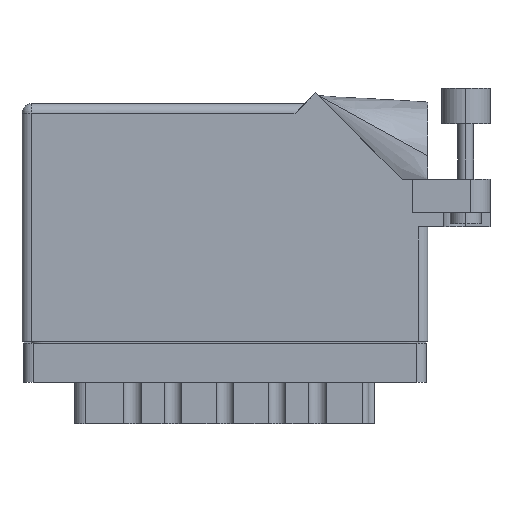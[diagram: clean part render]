
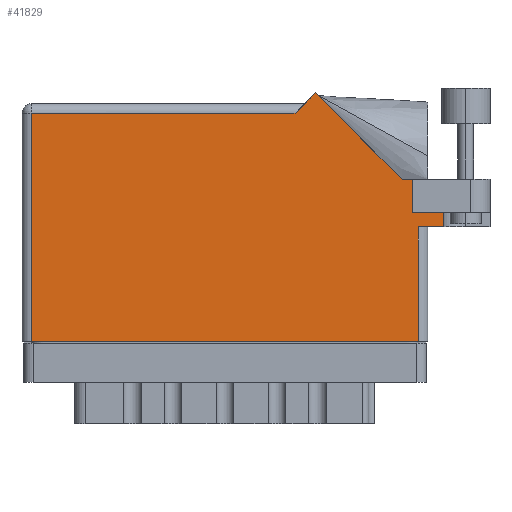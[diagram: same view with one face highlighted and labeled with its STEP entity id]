
A CAD part, front view. The second image highlights one B-rep face of the part: STEP entity #41829.
In plain terms, the highlighted face is planar.
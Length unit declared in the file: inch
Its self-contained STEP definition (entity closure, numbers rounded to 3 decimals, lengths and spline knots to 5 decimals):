
#78 = DIRECTION ( 'NONE',  ( 0., 1., 0. ) ) ;
#1935 = LINE ( 'NONE', #53545, #23391 ) ;
#1975 = LINE ( 'NONE', #14312, #14341 ) ;
#2028 = LINE ( 'NONE', #33242, #18279 ) ;
#2442 = DIRECTION ( 'NONE',  ( -0.707, -0.707, 0. ) ) ;
#4687 = PLANE ( 'NONE',  #38663 ) ;
#5267 = CARTESIAN_POINT ( 'NONE',  ( 0., 1.468, 0. ) ) ;
#6086 = ORIENTED_EDGE ( 'NONE', *, *, #46386, .T. ) ;
#6422 = EDGE_CURVE ( 'NONE', #45393, #26172, #22502, .T. ) ;
#6703 = VERTEX_POINT ( 'NONE', #28338 ) ;
#7091 = DIRECTION ( 'NONE',  ( 0., -1., 0. ) ) ;
#8161 = CARTESIAN_POINT ( 'NONE',  ( 0., 0., 0. ) ) ;
#8495 = DIRECTION ( 'NONE',  ( -1., 0., 0. ) ) ;
#11609 = CARTESIAN_POINT ( 'NONE',  ( 2.7135, 1.16177, 0. ) ) ;
#12663 = CARTESIAN_POINT ( 'NONE',  ( 0., 1.53, 0. ) ) ;
#12976 = CARTESIAN_POINT ( 'NONE',  ( 0.062, 0., 0. ) ) ;
#13399 = ORIENTED_EDGE ( 'NONE', *, *, #14437, .F. ) ;
#14090 = VECTOR ( 'NONE', #7091, 39.37008 ) ;
#14312 = CARTESIAN_POINT ( 'NONE',  ( 0.062, 0., 0. ) ) ;
#14341 = VECTOR ( 'NONE', #22461, 39.37008 ) ;
#14437 = EDGE_CURVE ( 'NONE', #32994, #45393, #21769, .T. ) ;
#14681 = CARTESIAN_POINT ( 'NONE',  ( 2.512, 0.831, 0. ) ) ;
#14711 = VECTOR ( 'NONE', #39301, 39.37008 ) ;
#15685 = VECTOR ( 'NONE', #33234, 39.37008 ) ;
#16981 = LINE ( 'NONE', #8161, #15685 ) ;
#17054 = DIRECTION ( 'NONE',  ( -1., 0., 0. ) ) ;
#18279 = VECTOR ( 'NONE', #49422, 39.37008 ) ;
#18622 = VECTOR ( 'NONE', #78, 39.37008 ) ;
#18752 = CARTESIAN_POINT ( 'NONE',  ( 2.512, 1.044, 0. ) ) ;
#21435 = CARTESIAN_POINT ( 'NONE',  ( 2.44642, 1.044, 0. ) ) ;
#21507 = EDGE_CURVE ( 'NONE', #52375, #6703, #31253, .T. ) ;
#21769 = LINE ( 'NONE', #46541, #53081 ) ;
#22461 = DIRECTION ( 'NONE',  ( 0., -1., 0. ) ) ;
#22496 = VERTEX_POINT ( 'NONE', #32623 ) ;
#22502 = LINE ( 'NONE', #11609, #14090 ) ;
#22511 = LINE ( 'NONE', #37193, #18622 ) ;
#23029 = FACE_OUTER_BOUND ( 'NONE', #51310, .T. ) ;
#23140 = ORIENTED_EDGE ( 'NONE', *, *, #25899, .T. ) ;
#23391 = VECTOR ( 'NONE', #2442, 39.37008 ) ;
#23693 = CARTESIAN_POINT ( 'NONE',  ( 2.7135, 0.831, 0. ) ) ;
#23819 = CARTESIAN_POINT ( 'NONE',  ( 2.44642, 1.044, 0. ) ) ;
#23852 = CARTESIAN_POINT ( 'NONE',  ( 1.757, 1.468, 0. ) ) ;
#24695 = CARTESIAN_POINT ( 'NONE',  ( 2.55, 0.737, 0. ) ) ;
#24948 = VERTEX_POINT ( 'NONE', #24695 ) ;
#25200 = DIRECTION ( 'NONE',  ( 0., 0., -1. ) ) ;
#25675 = VECTOR ( 'NONE', #35914, 39.37008 ) ;
#25816 = VERTEX_POINT ( 'NONE', #39876 ) ;
#25899 = EDGE_CURVE ( 'NONE', #26541, #31645, #38672, .T. ) ;
#26172 = VERTEX_POINT ( 'NONE', #37884 ) ;
#26541 = VERTEX_POINT ( 'NONE', #18752 ) ;
#26849 = ORIENTED_EDGE ( 'NONE', *, *, #43912, .T. ) ;
#26880 = EDGE_CURVE ( 'NONE', #31645, #22496, #49626, .T. ) ;
#27528 = ORIENTED_EDGE ( 'NONE', *, *, #6422, .F. ) ;
#28338 = CARTESIAN_POINT ( 'NONE',  ( 0.062, 1.468, 0. ) ) ;
#28623 = VECTOR ( 'NONE', #17054, 39.37008 ) ;
#29414 = VECTOR ( 'NONE', #29619, 39.37008 ) ;
#29619 = DIRECTION ( 'NONE',  ( -0.707, 0.707, 0. ) ) ;
#31253 = LINE ( 'NONE', #5267, #28623 ) ;
#31645 = VERTEX_POINT ( 'NONE', #23819 ) ;
#32078 = ORIENTED_EDGE ( 'NONE', *, *, #37464, .T. ) ;
#32623 = CARTESIAN_POINT ( 'NONE',  ( 1.88971, 1.60071, 0. ) ) ;
#32932 = LINE ( 'NONE', #46960, #14711 ) ;
#32994 = VERTEX_POINT ( 'NONE', #14681 ) ;
#33209 = EDGE_CURVE ( 'NONE', #32994, #26541, #22511, .T. ) ;
#33234 = DIRECTION ( 'NONE',  ( 1., 0., 0. ) ) ;
#33242 = CARTESIAN_POINT ( 'NONE',  ( 2.55, 0.737, 0. ) ) ;
#33291 = DIRECTION ( 'NONE',  ( 1., 0., 0. ) ) ;
#34395 = ORIENTED_EDGE ( 'NONE', *, *, #43591, .T. ) ;
#35914 = DIRECTION ( 'NONE',  ( -1., 0., 0. ) ) ;
#37193 = CARTESIAN_POINT ( 'NONE',  ( 2.512, 0.831, 0. ) ) ;
#37434 = ORIENTED_EDGE ( 'NONE', *, *, #53587, .T. ) ;
#37464 = EDGE_CURVE ( 'NONE', #22496, #52375, #1935, .T. ) ;
#37884 = CARTESIAN_POINT ( 'NONE',  ( 2.7135, 0.737, 0. ) ) ;
#38266 = ORIENTED_EDGE ( 'NONE', *, *, #33209, .T. ) ;
#38663 = AXIS2_PLACEMENT_3D ( 'NONE', #12663, #25200, #8495 ) ;
#38672 = LINE ( 'NONE', #40570, #25675 ) ;
#39301 = DIRECTION ( 'NONE',  ( 1., 0., 0. ) ) ;
#39876 = CARTESIAN_POINT ( 'NONE',  ( 2.55, 0., 0. ) ) ;
#40570 = CARTESIAN_POINT ( 'NONE',  ( 3.012, 1.044, 0. ) ) ;
#41829 = ADVANCED_FACE ( 'NONE', ( #23029 ), #4687, .F. ) ;
#42380 = VERTEX_POINT ( 'NONE', #12976 ) ;
#43591 = EDGE_CURVE ( 'NONE', #25816, #24948, #2028, .T. ) ;
#43912 = EDGE_CURVE ( 'NONE', #6703, #42380, #1975, .T. ) ;
#44953 = ORIENTED_EDGE ( 'NONE', *, *, #26880, .T. ) ;
#45393 = VERTEX_POINT ( 'NONE', #23693 ) ;
#46386 = EDGE_CURVE ( 'NONE', #24948, #26172, #32932, .T. ) ;
#46541 = CARTESIAN_POINT ( 'NONE',  ( 2.512, 0.831, 0. ) ) ;
#46960 = CARTESIAN_POINT ( 'NONE',  ( 2.612, 0.737, 0. ) ) ;
#49422 = DIRECTION ( 'NONE',  ( 0., 1., 0. ) ) ;
#49626 = LINE ( 'NONE', #21435, #29414 ) ;
#51310 = EDGE_LOOP ( 'NONE', ( #37434, #34395, #6086, #27528, #13399, #38266, #23140, #44953, #32078, #51864, #26849 ) ) ;
#51864 = ORIENTED_EDGE ( 'NONE', *, *, #21507, .T. ) ;
#52375 = VERTEX_POINT ( 'NONE', #23852 ) ;
#53081 = VECTOR ( 'NONE', #33291, 39.37008 ) ;
#53545 = CARTESIAN_POINT ( 'NONE',  ( 1.819, 1.53, 0. ) ) ;
#53587 = EDGE_CURVE ( 'NONE', #42380, #25816, #16981, .T. ) ;
